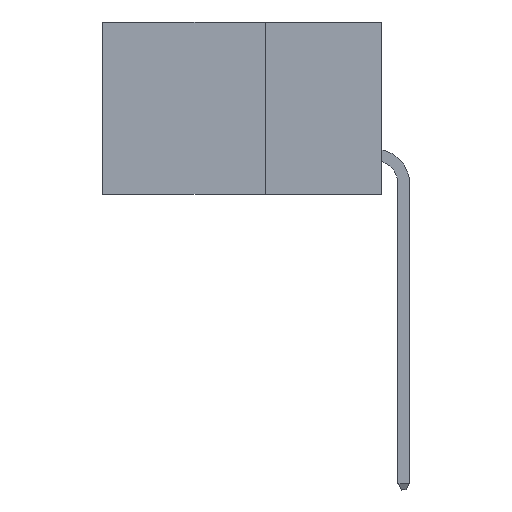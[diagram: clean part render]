
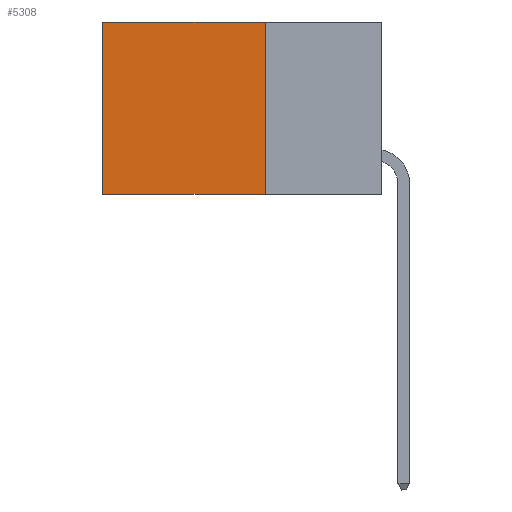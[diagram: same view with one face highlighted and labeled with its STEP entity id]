
A CAD part, left-side view. The second image highlights one B-rep face of the part: STEP entity #5308.
In plain terms, the highlighted planar face has unit normal (-1, 0, 0).
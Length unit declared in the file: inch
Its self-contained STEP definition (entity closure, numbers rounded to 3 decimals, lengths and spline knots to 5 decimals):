
#144 = DIRECTION ( 'NONE',  ( 0., 1., 0. ) ) ;
#772 = ORIENTED_EDGE ( 'NONE', *, *, #14327, .T. ) ;
#1120 = CARTESIAN_POINT ( 'NONE',  ( 0.2875, 0.25, 0. ) ) ;
#2639 = VERTEX_POINT ( 'NONE', #1120 ) ;
#2746 = DIRECTION ( 'NONE',  ( 0., 1., 0. ) ) ;
#3589 = VECTOR ( 'NONE', #144, 39.37008 ) ;
#3701 = VERTEX_POINT ( 'NONE', #14792 ) ;
#3816 = EDGE_LOOP ( 'NONE', ( #772, #16659, #14271, #6676 ) ) ;
#4213 = CARTESIAN_POINT ( 'NONE',  ( 0.2875, 0.6, 0. ) ) ;
#4510 = VERTEX_POINT ( 'NONE', #9993 ) ;
#4517 = EDGE_CURVE ( 'NONE', #2639, #3701, #8330, .T. ) ;
#4649 = VECTOR ( 'NONE', #6203, 39.37008 ) ;
#4829 = CARTESIAN_POINT ( 'NONE',  ( 0.2875, 0.25, 0. ) ) ;
#5006 = EDGE_CURVE ( 'NONE', #2639, #10838, #10506, .T. ) ;
#5013 = DIRECTION ( 'NONE',  ( 1., 0., 0. ) ) ;
#5308 = ADVANCED_FACE ( 'NONE', ( #13766 ), #16447, .F. ) ;
#6203 = DIRECTION ( 'NONE',  ( 0., 0., -1. ) ) ;
#6676 = ORIENTED_EDGE ( 'NONE', *, *, #5006, .T. ) ;
#8330 = LINE ( 'NONE', #15187, #4649 ) ;
#9167 = AXIS2_PLACEMENT_3D ( 'NONE', #16555, #5013, #10069 ) ;
#9993 = CARTESIAN_POINT ( 'NONE',  ( 0.2875, 0.6, -0.37 ) ) ;
#10069 = DIRECTION ( 'NONE',  ( 0., 0., -1. ) ) ;
#10506 = LINE ( 'NONE', #4829, #3589 ) ;
#10838 = VERTEX_POINT ( 'NONE', #4213 ) ;
#12007 = DIRECTION ( 'NONE',  ( 0., 0., -1. ) ) ;
#12939 = VECTOR ( 'NONE', #2746, 39.37008 ) ;
#13330 = LINE ( 'NONE', #15821, #12939 ) ;
#13637 = VECTOR ( 'NONE', #12007, 39.37008 ) ;
#13766 = FACE_OUTER_BOUND ( 'NONE', #3816, .T. ) ;
#14271 = ORIENTED_EDGE ( 'NONE', *, *, #4517, .F. ) ;
#14327 = EDGE_CURVE ( 'NONE', #10838, #4510, #16682, .T. ) ;
#14792 = CARTESIAN_POINT ( 'NONE',  ( 0.2875, 0.25, -0.37 ) ) ;
#15187 = CARTESIAN_POINT ( 'NONE',  ( 0.2875, 0.25, 0. ) ) ;
#15821 = CARTESIAN_POINT ( 'NONE',  ( 0.2875, 0.25, -0.37 ) ) ;
#15928 = CARTESIAN_POINT ( 'NONE',  ( 0.2875, 0.6, 0. ) ) ;
#16447 = PLANE ( 'NONE',  #9167 ) ;
#16555 = CARTESIAN_POINT ( 'NONE',  ( 0.2875, 0.25, 0. ) ) ;
#16659 = ORIENTED_EDGE ( 'NONE', *, *, #16819, .F. ) ;
#16682 = LINE ( 'NONE', #15928, #13637 ) ;
#16819 = EDGE_CURVE ( 'NONE', #3701, #4510, #13330, .T. ) ;
